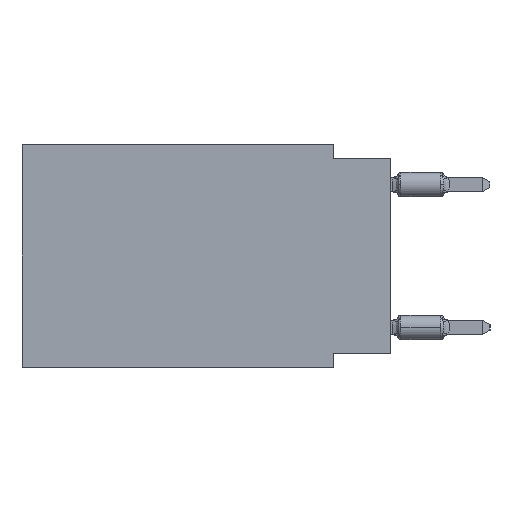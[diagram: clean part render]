
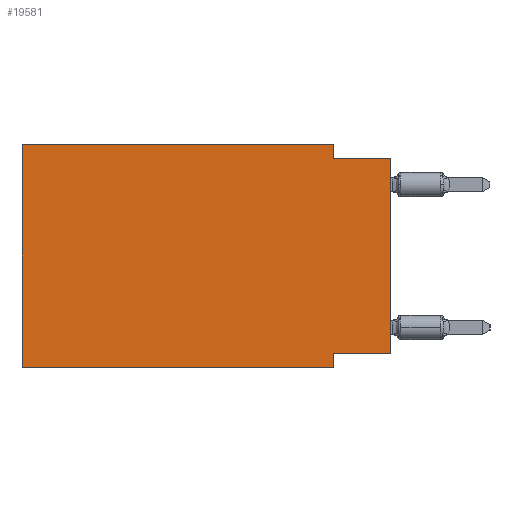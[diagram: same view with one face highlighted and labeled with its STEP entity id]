
A CAD part, left-side view. The second image highlights one B-rep face of the part: STEP entity #19581.
In plain terms, the highlighted planar face has unit normal (-1, 0, 0).
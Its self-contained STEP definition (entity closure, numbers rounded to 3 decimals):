
#345 = LINE ( 'NONE', #12674, #16772 ) ;
#601 = ORIENTED_EDGE ( 'NONE', *, *, #6655, .T. ) ;
#913 = VERTEX_POINT ( 'NONE', #4678 ) ;
#958 = EDGE_CURVE ( 'NONE', #15519, #6266, #1764, .T. ) ;
#1221 = VECTOR ( 'NONE', #5590, 1000. ) ;
#1764 = LINE ( 'NONE', #3159, #3982 ) ;
#2028 = CARTESIAN_POINT ( 'NONE',  ( 0., 0., -9.271 ) ) ;
#2073 = VECTOR ( 'NONE', #19871, 1000. ) ;
#2296 = VERTEX_POINT ( 'NONE', #2028 ) ;
#2360 = CARTESIAN_POINT ( 'NONE',  ( 0., 16.383, -9.906 ) ) ;
#3159 = CARTESIAN_POINT ( 'NONE',  ( 0., 2.54, 0. ) ) ;
#3982 = VECTOR ( 'NONE', #22499, 1000. ) ;
#4252 = VECTOR ( 'NONE', #17254, 1000. ) ;
#4490 = LINE ( 'NONE', #21768, #15228 ) ;
#4539 = DIRECTION ( 'NONE',  ( 0., 0., 1. ) ) ;
#4678 = CARTESIAN_POINT ( 'NONE',  ( 0., 2.54, -9.271 ) ) ;
#4755 = VERTEX_POINT ( 'NONE', #18157 ) ;
#5040 = CARTESIAN_POINT ( 'NONE',  ( 0., 16.383, 0. ) ) ;
#5590 = DIRECTION ( 'NONE',  ( 0., -1., 0. ) ) ;
#5984 = DIRECTION ( 'NONE',  ( 0., -1., 0. ) ) ;
#6266 = VERTEX_POINT ( 'NONE', #9179 ) ;
#6493 = CARTESIAN_POINT ( 'NONE',  ( 0., 0., -9.271 ) ) ;
#6655 = EDGE_CURVE ( 'NONE', #2296, #15502, #17089, .T. ) ;
#6664 = CARTESIAN_POINT ( 'NONE',  ( 0., 16.383, 0. ) ) ;
#7047 = CARTESIAN_POINT ( 'NONE',  ( 0., 16.383, -9.906 ) ) ;
#7541 = CARTESIAN_POINT ( 'NONE',  ( 0., 16.383, 0. ) ) ;
#8349 = CARTESIAN_POINT ( 'NONE',  ( 0., 0., 0. ) ) ;
#8802 = ORIENTED_EDGE ( 'NONE', *, *, #18591, .F. ) ;
#8993 = DIRECTION ( 'NONE',  ( 0., 0., -1. ) ) ;
#9179 = CARTESIAN_POINT ( 'NONE',  ( 0., 2.54, -0.635 ) ) ;
#9183 = LINE ( 'NONE', #2360, #1221 ) ;
#9681 = DIRECTION ( 'NONE',  ( 0., 0., -1. ) ) ;
#10246 = ORIENTED_EDGE ( 'NONE', *, *, #20189, .F. ) ;
#10362 = EDGE_CURVE ( 'NONE', #13277, #4755, #21710, .T. ) ;
#10437 = ORIENTED_EDGE ( 'NONE', *, *, #15423, .F. ) ;
#10883 = AXIS2_PLACEMENT_3D ( 'NONE', #6664, #13366, #9681 ) ;
#11861 = EDGE_CURVE ( 'NONE', #2296, #913, #17079, .T. ) ;
#11908 = ORIENTED_EDGE ( 'NONE', *, *, #10362, .F. ) ;
#12175 = LINE ( 'NONE', #5040, #4252 ) ;
#12674 = CARTESIAN_POINT ( 'NONE',  ( 0., 2.54, -9.906 ) ) ;
#12779 = EDGE_LOOP ( 'NONE', ( #601, #8802, #15464, #10246, #11908, #16207, #10437, #15801 ) ) ;
#13277 = VERTEX_POINT ( 'NONE', #7047 ) ;
#13366 = DIRECTION ( 'NONE',  ( 1., 0., 0. ) ) ;
#13599 = PLANE ( 'NONE',  #10883 ) ;
#14626 = VECTOR ( 'NONE', #15565, 1000. ) ;
#14970 = CARTESIAN_POINT ( 'NONE',  ( 0., 0., -0.635 ) ) ;
#15228 = VECTOR ( 'NONE', #5984, 1000. ) ;
#15423 = EDGE_CURVE ( 'NONE', #913, #15693, #345, .T. ) ;
#15464 = ORIENTED_EDGE ( 'NONE', *, *, #958, .F. ) ;
#15502 = VERTEX_POINT ( 'NONE', #14970 ) ;
#15519 = VERTEX_POINT ( 'NONE', #18762 ) ;
#15565 = DIRECTION ( 'NONE',  ( 0., 1., 0. ) ) ;
#15693 = VERTEX_POINT ( 'NONE', #17607 ) ;
#15801 = ORIENTED_EDGE ( 'NONE', *, *, #11861, .F. ) ;
#16207 = ORIENTED_EDGE ( 'NONE', *, *, #17557, .T. ) ;
#16772 = VECTOR ( 'NONE', #8993, 1000. ) ;
#17042 = FACE_OUTER_BOUND ( 'NONE', #12779, .T. ) ;
#17079 = LINE ( 'NONE', #6493, #14626 ) ;
#17089 = LINE ( 'NONE', #8349, #22646 ) ;
#17254 = DIRECTION ( 'NONE',  ( 0., -1., 0. ) ) ;
#17557 = EDGE_CURVE ( 'NONE', #13277, #15693, #9183, .T. ) ;
#17607 = CARTESIAN_POINT ( 'NONE',  ( 0., 2.54, -9.906 ) ) ;
#18157 = CARTESIAN_POINT ( 'NONE',  ( 0., 16.383, 0. ) ) ;
#18591 = EDGE_CURVE ( 'NONE', #6266, #15502, #4490, .T. ) ;
#18762 = CARTESIAN_POINT ( 'NONE',  ( 0., 2.54, 0. ) ) ;
#19581 = ADVANCED_FACE ( 'NONE', ( #17042 ), #13599, .F. ) ;
#19871 = DIRECTION ( 'NONE',  ( 0., 0., 1. ) ) ;
#20189 = EDGE_CURVE ( 'NONE', #4755, #15519, #12175, .T. ) ;
#21710 = LINE ( 'NONE', #7541, #2073 ) ;
#21768 = CARTESIAN_POINT ( 'NONE',  ( 0., 0., -0.635 ) ) ;
#22499 = DIRECTION ( 'NONE',  ( 0., 0., -1. ) ) ;
#22646 = VECTOR ( 'NONE', #4539, 1000. ) ;
